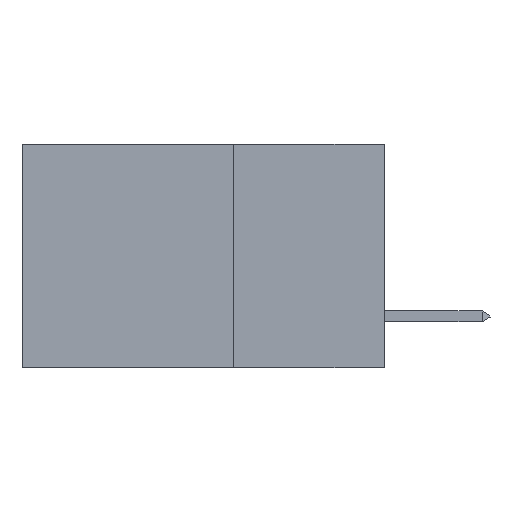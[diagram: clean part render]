
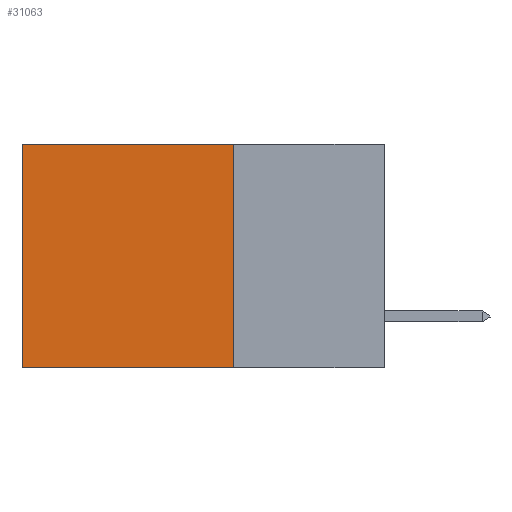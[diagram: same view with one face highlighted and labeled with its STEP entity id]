
A CAD part, left-side view. The second image highlights one B-rep face of the part: STEP entity #31063.
In plain terms, the highlighted planar face has unit normal (-1, 0, 0).
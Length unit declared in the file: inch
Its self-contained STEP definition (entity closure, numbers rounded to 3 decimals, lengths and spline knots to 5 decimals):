
#63 = EDGE_CURVE ( 'NONE', #5131, #1620, #5958, .T. ) ;
#280 = PLANE ( 'NONE',  #28834 ) ;
#1620 = VERTEX_POINT ( 'NONE', #29637 ) ;
#2694 = CARTESIAN_POINT ( 'NONE',  ( 0.2875, 0.6, 0. ) ) ;
#3520 = VERTEX_POINT ( 'NONE', #27094 ) ;
#3697 = ORIENTED_EDGE ( 'NONE', *, *, #34373, .T. ) ;
#4017 = VECTOR ( 'NONE', #10741, 39.37008 ) ;
#4907 = ORIENTED_EDGE ( 'NONE', *, *, #63, .F. ) ;
#5131 = VERTEX_POINT ( 'NONE', #27519 ) ;
#5723 = EDGE_LOOP ( 'NONE', ( #7939, #32149, #4907, #3697 ) ) ;
#5830 = DIRECTION ( 'NONE',  ( 0., 0., -1. ) ) ;
#5958 = LINE ( 'NONE', #11542, #20542 ) ;
#7939 = ORIENTED_EDGE ( 'NONE', *, *, #25673, .T. ) ;
#8020 = CARTESIAN_POINT ( 'NONE',  ( 0.2875, 0.25, -0.37 ) ) ;
#10741 = DIRECTION ( 'NONE',  ( 0., 1., 0. ) ) ;
#11542 = CARTESIAN_POINT ( 'NONE',  ( 0.2875, 0.25, 0. ) ) ;
#11738 = EDGE_CURVE ( 'NONE', #1620, #3520, #24540, .T. ) ;
#13042 = FACE_OUTER_BOUND ( 'NONE', #5723, .T. ) ;
#16934 = DIRECTION ( 'NONE',  ( 0., 0., -1. ) ) ;
#18106 = VERTEX_POINT ( 'NONE', #2694 ) ;
#18333 = DIRECTION ( 'NONE',  ( 0., 1., 0. ) ) ;
#19534 = DIRECTION ( 'NONE',  ( 0., 0., -1. ) ) ;
#20542 = VECTOR ( 'NONE', #16934, 39.37008 ) ;
#24540 = LINE ( 'NONE', #8020, #4017 ) ;
#24723 = DIRECTION ( 'NONE',  ( 1., 0., 0. ) ) ;
#25673 = EDGE_CURVE ( 'NONE', #18106, #3520, #27690, .T. ) ;
#27094 = CARTESIAN_POINT ( 'NONE',  ( 0.2875, 0.6, -0.37 ) ) ;
#27369 = CARTESIAN_POINT ( 'NONE',  ( 0.2875, 0.25, 0. ) ) ;
#27519 = CARTESIAN_POINT ( 'NONE',  ( 0.2875, 0.25, 0. ) ) ;
#27690 = LINE ( 'NONE', #33273, #32445 ) ;
#28834 = AXIS2_PLACEMENT_3D ( 'NONE', #27369, #24723, #5830 ) ;
#29505 = VECTOR ( 'NONE', #18333, 39.37008 ) ;
#29637 = CARTESIAN_POINT ( 'NONE',  ( 0.2875, 0.25, -0.37 ) ) ;
#31063 = ADVANCED_FACE ( 'NONE', ( #13042 ), #280, .F. ) ;
#32149 = ORIENTED_EDGE ( 'NONE', *, *, #11738, .F. ) ;
#32298 = CARTESIAN_POINT ( 'NONE',  ( 0.2875, 0.25, 0. ) ) ;
#32445 = VECTOR ( 'NONE', #19534, 39.37008 ) ;
#33273 = CARTESIAN_POINT ( 'NONE',  ( 0.2875, 0.6, 0. ) ) ;
#34373 = EDGE_CURVE ( 'NONE', #5131, #18106, #35056, .T. ) ;
#35056 = LINE ( 'NONE', #32298, #29505 ) ;
